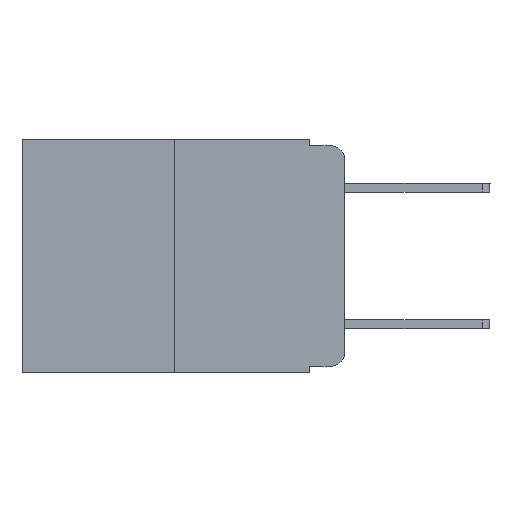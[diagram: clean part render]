
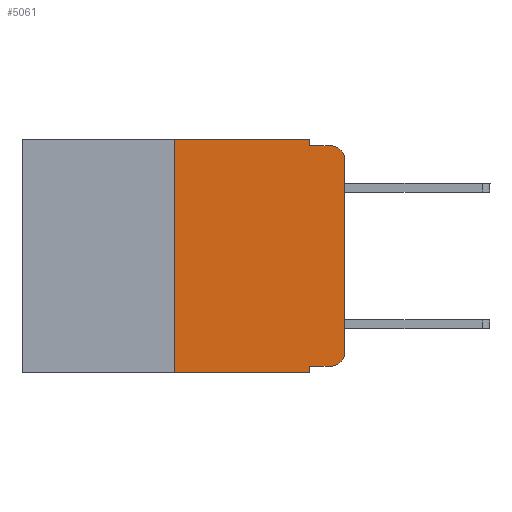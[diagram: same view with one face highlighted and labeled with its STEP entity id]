
A CAD part, left-side view. The second image highlights one B-rep face of the part: STEP entity #5061.
In plain terms, the highlighted planar face has unit normal (-1, 0, 0).
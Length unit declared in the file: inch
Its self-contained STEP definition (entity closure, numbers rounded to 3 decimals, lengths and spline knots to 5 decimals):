
#16 = ORIENTED_EDGE ( 'NONE', *, *, #25435, .F. ) ;
#119 = LINE ( 'NONE', #7582, #3743 ) ;
#330 = CARTESIAN_POINT ( 'NONE',  ( 0., 0.051, 0. ) ) ;
#552 = ORIENTED_EDGE ( 'NONE', *, *, #12535, .F. ) ;
#662 = CARTESIAN_POINT ( 'NONE',  ( 0., 0.02, -0.333 ) ) ;
#1839 = VERTEX_POINT ( 'NONE', #15504 ) ;
#1924 = DIRECTION ( 'NONE',  ( 0., -1., 0. ) ) ;
#2171 = LINE ( 'NONE', #5907, #12754 ) ;
#2556 = CARTESIAN_POINT ( 'NONE',  ( 0., 0.02, -0.01 ) ) ;
#2656 = CARTESIAN_POINT ( 'NONE',  ( 0., 0., -0.03 ) ) ;
#2698 = VERTEX_POINT ( 'NONE', #24379 ) ;
#2834 = CARTESIAN_POINT ( 'NONE',  ( 0., 0.25, -0.343 ) ) ;
#2945 = DIRECTION ( 'NONE',  ( 0., -1., 0. ) ) ;
#3299 = LINE ( 'NONE', #23285, #21855 ) ;
#3300 = ORIENTED_EDGE ( 'NONE', *, *, #9566, .T. ) ;
#3487 = CARTESIAN_POINT ( 'NONE',  ( 0., 0.051, -0.01 ) ) ;
#3743 = VECTOR ( 'NONE', #4233, 39.37008 ) ;
#4233 = DIRECTION ( 'NONE',  ( 0., -1., 0. ) ) ;
#4387 = CARTESIAN_POINT ( 'NONE',  ( 0., 0.02, -0.03 ) ) ;
#4456 = DIRECTION ( 'NONE',  ( 0., 0., -1. ) ) ;
#4667 = DIRECTION ( 'NONE',  ( 0., 0., -1. ) ) ;
#5061 = ADVANCED_FACE ( 'NONE', ( #13571 ), #5713, .F. ) ;
#5713 = PLANE ( 'NONE',  #7290 ) ;
#5894 = ORIENTED_EDGE ( 'NONE', *, *, #11683, .F. ) ;
#5907 = CARTESIAN_POINT ( 'NONE',  ( 0., 0., 0. ) ) ;
#6072 = DIRECTION ( 'NONE',  ( -1., 0., 0. ) ) ;
#6160 = DIRECTION ( 'NONE',  ( 0., 0., 1. ) ) ;
#6250 = LINE ( 'NONE', #8311, #7334 ) ;
#6305 = DIRECTION ( 'NONE',  ( 0., 0., 1. ) ) ;
#6389 = VERTEX_POINT ( 'NONE', #2556 ) ;
#6880 = CARTESIAN_POINT ( 'NONE',  ( 0., 0.051, 0. ) ) ;
#7290 = AXIS2_PLACEMENT_3D ( 'NONE', #7384, #24958, #15643 ) ;
#7334 = VECTOR ( 'NONE', #4456, 39.37008 ) ;
#7384 = CARTESIAN_POINT ( 'NONE',  ( 0., 0.473, 0. ) ) ;
#7570 = EDGE_CURVE ( 'NONE', #18259, #10095, #2171, .T. ) ;
#7582 = CARTESIAN_POINT ( 'NONE',  ( 0., 0.051, -0.333 ) ) ;
#8311 = CARTESIAN_POINT ( 'NONE',  ( 0., 0.051, 0. ) ) ;
#8635 = DIRECTION ( 'NONE',  ( -1., 0., 0. ) ) ;
#9566 = EDGE_CURVE ( 'NONE', #18661, #11783, #3299, .T. ) ;
#9781 = ORIENTED_EDGE ( 'NONE', *, *, #18729, .F. ) ;
#9975 = EDGE_LOOP ( 'NONE', ( #18104, #14263, #552, #5894, #16, #9781, #3300, #19203, #22179, #19598 ) ) ;
#10095 = VERTEX_POINT ( 'NONE', #2656 ) ;
#11213 = LINE ( 'NONE', #3487, #20329 ) ;
#11683 = EDGE_CURVE ( 'NONE', #19229, #1839, #21859, .T. ) ;
#11783 = VERTEX_POINT ( 'NONE', #14098 ) ;
#12291 = EDGE_CURVE ( 'NONE', #18693, #18259, #13312, .T. ) ;
#12535 = EDGE_CURVE ( 'NONE', #1839, #6389, #11213, .T. ) ;
#12737 = LINE ( 'NONE', #20624, #25194 ) ;
#12754 = VECTOR ( 'NONE', #6160, 39.37008 ) ;
#12767 = CARTESIAN_POINT ( 'NONE',  ( 0., 0.25, 0. ) ) ;
#13312 = CIRCLE ( 'NONE', #19918, 0.02 ) ;
#13571 = FACE_OUTER_BOUND ( 'NONE', #9975, .T. ) ;
#14039 = CIRCLE ( 'NONE', #16089, 0.02 ) ;
#14067 = CARTESIAN_POINT ( 'NONE',  ( 0., 0.02, -0.313 ) ) ;
#14098 = CARTESIAN_POINT ( 'NONE',  ( 0., 0.051, -0.343 ) ) ;
#14155 = DIRECTION ( 'NONE',  ( 0., -1., 0. ) ) ;
#14263 = ORIENTED_EDGE ( 'NONE', *, *, #23670, .T. ) ;
#14437 = LINE ( 'NONE', #23994, #23802 ) ;
#14443 = DIRECTION ( 'NONE',  ( 0., 0., -1. ) ) ;
#14850 = CARTESIAN_POINT ( 'NONE',  ( 0., 0., -0.313 ) ) ;
#15504 = CARTESIAN_POINT ( 'NONE',  ( 0., 0.051, -0.01 ) ) ;
#15643 = DIRECTION ( 'NONE',  ( 0., 0., -1. ) ) ;
#16089 = AXIS2_PLACEMENT_3D ( 'NONE', #4387, #8635, #14443 ) ;
#18104 = ORIENTED_EDGE ( 'NONE', *, *, #7570, .T. ) ;
#18259 = VERTEX_POINT ( 'NONE', #14850 ) ;
#18661 = VERTEX_POINT ( 'NONE', #2834 ) ;
#18693 = VERTEX_POINT ( 'NONE', #662 ) ;
#18729 = EDGE_CURVE ( 'NONE', #18661, #21292, #14437, .T. ) ;
#19203 = ORIENTED_EDGE ( 'NONE', *, *, #20913, .F. ) ;
#19229 = VERTEX_POINT ( 'NONE', #6880 ) ;
#19598 = ORIENTED_EDGE ( 'NONE', *, *, #12291, .T. ) ;
#19918 = AXIS2_PLACEMENT_3D ( 'NONE', #14067, #6072, #4667 ) ;
#20329 = VECTOR ( 'NONE', #1924, 39.37008 ) ;
#20624 = CARTESIAN_POINT ( 'NONE',  ( 0., 0.473, 0. ) ) ;
#20913 = EDGE_CURVE ( 'NONE', #2698, #11783, #6250, .T. ) ;
#21292 = VERTEX_POINT ( 'NONE', #12767 ) ;
#21855 = VECTOR ( 'NONE', #14155, 39.37008 ) ;
#21859 = LINE ( 'NONE', #330, #24433 ) ;
#22179 = ORIENTED_EDGE ( 'NONE', *, *, #23931, .T. ) ;
#23285 = CARTESIAN_POINT ( 'NONE',  ( 0., 0.473, -0.343 ) ) ;
#23670 = EDGE_CURVE ( 'NONE', #10095, #6389, #14039, .T. ) ;
#23802 = VECTOR ( 'NONE', #6305, 39.37008 ) ;
#23931 = EDGE_CURVE ( 'NONE', #2698, #18693, #119, .T. ) ;
#23994 = CARTESIAN_POINT ( 'NONE',  ( 0., 0.25, 0. ) ) ;
#24307 = DIRECTION ( 'NONE',  ( 0., 0., -1. ) ) ;
#24379 = CARTESIAN_POINT ( 'NONE',  ( 0., 0.051, -0.333 ) ) ;
#24433 = VECTOR ( 'NONE', #24307, 39.37008 ) ;
#24958 = DIRECTION ( 'NONE',  ( 1., 0., 0. ) ) ;
#25194 = VECTOR ( 'NONE', #2945, 39.37008 ) ;
#25435 = EDGE_CURVE ( 'NONE', #21292, #19229, #12737, .T. ) ;
